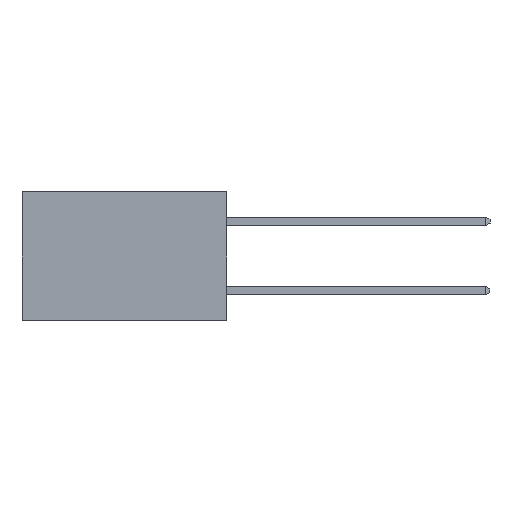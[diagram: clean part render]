
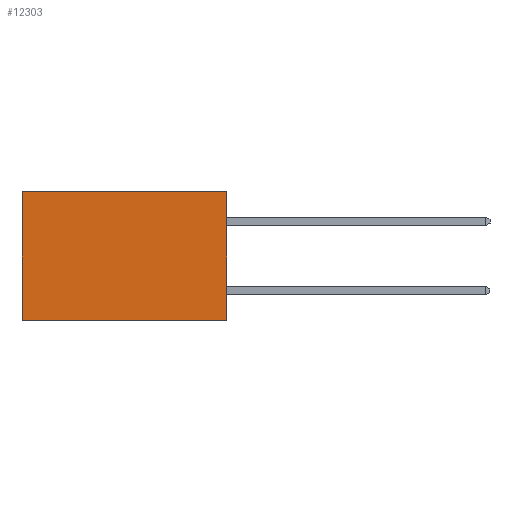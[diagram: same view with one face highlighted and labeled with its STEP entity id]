
A CAD part, left-side view. The second image highlights one B-rep face of the part: STEP entity #12303.
In plain terms, the highlighted planar face has unit normal (-1, 0, 0).
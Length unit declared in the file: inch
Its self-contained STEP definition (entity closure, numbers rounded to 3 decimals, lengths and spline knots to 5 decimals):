
#231 = DIRECTION ( 'NONE',  ( 0., 1., 0. ) ) ;
#624 = CARTESIAN_POINT ( 'NONE',  ( 0.277, 0., -0.37 ) ) ;
#882 = LINE ( 'NONE', #2158, #17697 ) ;
#1037 = AXIS2_PLACEMENT_3D ( 'NONE', #17418, #17487, #7757 ) ;
#1101 = LINE ( 'NONE', #17333, #13589 ) ;
#1244 = CARTESIAN_POINT ( 'NONE',  ( 0.277, 0., -0.37 ) ) ;
#1359 = ORIENTED_EDGE ( 'NONE', *, *, #4950, .T. ) ;
#1707 = LINE ( 'NONE', #10148, #5607 ) ;
#1751 = VERTEX_POINT ( 'NONE', #7967 ) ;
#1877 = ORIENTED_EDGE ( 'NONE', *, *, #5363, .F. ) ;
#1898 = LINE ( 'NONE', #1244, #14371 ) ;
#2158 = CARTESIAN_POINT ( 'NONE',  ( 0.277, 0.59, -0.37 ) ) ;
#2280 = DIRECTION ( 'NONE',  ( 0., 0., -1. ) ) ;
#2330 = CARTESIAN_POINT ( 'NONE',  ( 0.277, 0.59, 0. ) ) ;
#4473 = CARTESIAN_POINT ( 'NONE',  ( 0.277, 0.59, -0.37 ) ) ;
#4950 = EDGE_CURVE ( 'NONE', #11058, #18196, #882, .T. ) ;
#5363 = EDGE_CURVE ( 'NONE', #18650, #18196, #1898, .T. ) ;
#5607 = VECTOR ( 'NONE', #6915, 39.37008 ) ;
#6143 = PLANE ( 'NONE',  #1037 ) ;
#6915 = DIRECTION ( 'NONE',  ( 0., 0., -1. ) ) ;
#7757 = DIRECTION ( 'NONE',  ( 0., 0., -1. ) ) ;
#7967 = CARTESIAN_POINT ( 'NONE',  ( 0.277, 0., 0. ) ) ;
#10148 = CARTESIAN_POINT ( 'NONE',  ( 0.277, 0., -0.37 ) ) ;
#10314 = EDGE_LOOP ( 'NONE', ( #1359, #1877, #19154, #11036 ) ) ;
#11036 = ORIENTED_EDGE ( 'NONE', *, *, #16119, .T. ) ;
#11058 = VERTEX_POINT ( 'NONE', #2330 ) ;
#12303 = ADVANCED_FACE ( 'NONE', ( #15551 ), #6143, .F. ) ;
#13589 = VECTOR ( 'NONE', #20595, 39.37008 ) ;
#14371 = VECTOR ( 'NONE', #231, 39.37008 ) ;
#15551 = FACE_OUTER_BOUND ( 'NONE', #10314, .T. ) ;
#16119 = EDGE_CURVE ( 'NONE', #1751, #11058, #1101, .T. ) ;
#17333 = CARTESIAN_POINT ( 'NONE',  ( 0.277, 0., 0. ) ) ;
#17418 = CARTESIAN_POINT ( 'NONE',  ( 0.277, 0., -0.37 ) ) ;
#17487 = DIRECTION ( 'NONE',  ( 1., 0., 0. ) ) ;
#17697 = VECTOR ( 'NONE', #2280, 39.37008 ) ;
#18196 = VERTEX_POINT ( 'NONE', #4473 ) ;
#18650 = VERTEX_POINT ( 'NONE', #624 ) ;
#19154 = ORIENTED_EDGE ( 'NONE', *, *, #19839, .F. ) ;
#19839 = EDGE_CURVE ( 'NONE', #1751, #18650, #1707, .T. ) ;
#20595 = DIRECTION ( 'NONE',  ( 0., 1., 0. ) ) ;
